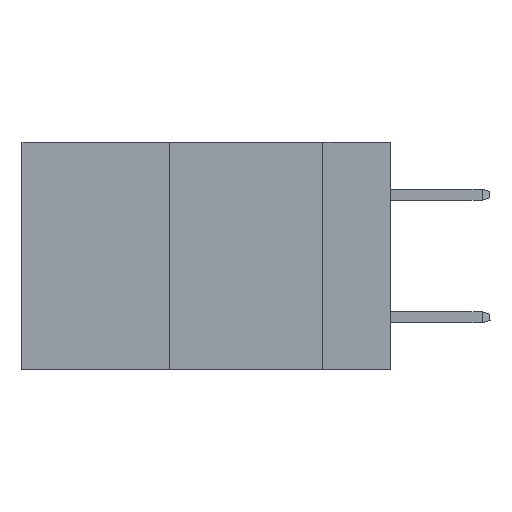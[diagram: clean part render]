
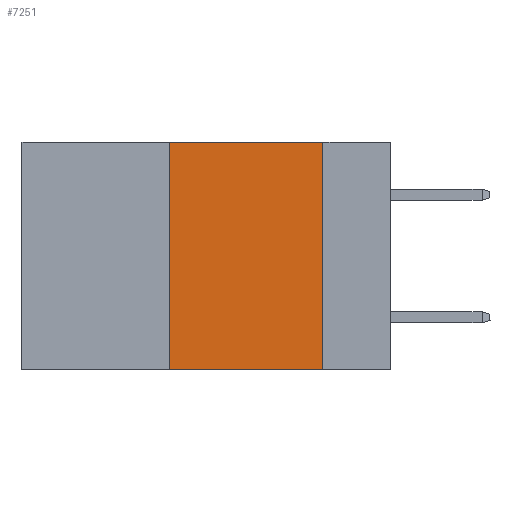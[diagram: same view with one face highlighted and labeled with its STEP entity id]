
A CAD part, left-side view. The second image highlights one B-rep face of the part: STEP entity #7251.
In plain terms, the highlighted planar face has unit normal (-1, 0, 0).
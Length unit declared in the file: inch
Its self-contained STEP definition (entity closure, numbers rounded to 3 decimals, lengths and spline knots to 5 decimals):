
#447 = EDGE_CURVE ( 'NONE', #14915, #10181, #13544, .T. ) ;
#807 = CARTESIAN_POINT ( 'NONE',  ( 0., 0.6, 0. ) ) ;
#812 = DIRECTION ( 'NONE',  ( 0., -1., 0. ) ) ;
#2126 = EDGE_LOOP ( 'NONE', ( #3064, #16125, #18472, #8523 ) ) ;
#2224 = DIRECTION ( 'NONE',  ( 1., 0., 0. ) ) ;
#2589 = DIRECTION ( 'NONE',  ( 0., -1., 0. ) ) ;
#3034 = DIRECTION ( 'NONE',  ( 0., 0., -1. ) ) ;
#3064 = ORIENTED_EDGE ( 'NONE', *, *, #12816, .F. ) ;
#3486 = CARTESIAN_POINT ( 'NONE',  ( 0., 0.6, -0.37 ) ) ;
#3496 = VECTOR ( 'NONE', #16801, 39.37008 ) ;
#3546 = EDGE_CURVE ( 'NONE', #14915, #8277, #7589, .T. ) ;
#4422 = VECTOR ( 'NONE', #812, 39.37008 ) ;
#6439 = LINE ( 'NONE', #11709, #15015 ) ;
#6639 = CARTESIAN_POINT ( 'NONE',  ( 0., 0.36, 0. ) ) ;
#7251 = ADVANCED_FACE ( 'NONE', ( #9905 ), #12539, .F. ) ;
#7589 = LINE ( 'NONE', #13075, #3496 ) ;
#8277 = VERTEX_POINT ( 'NONE', #6639 ) ;
#8523 = ORIENTED_EDGE ( 'NONE', *, *, #447, .T. ) ;
#8949 = CARTESIAN_POINT ( 'NONE',  ( 0., 0.36, -0.37 ) ) ;
#9905 = FACE_OUTER_BOUND ( 'NONE', #2126, .T. ) ;
#10031 = VERTEX_POINT ( 'NONE', #13288 ) ;
#10181 = VERTEX_POINT ( 'NONE', #11339 ) ;
#10905 = CARTESIAN_POINT ( 'NONE',  ( 0., 0.6, 0. ) ) ;
#11339 = CARTESIAN_POINT ( 'NONE',  ( 0., 0.11, -0.37 ) ) ;
#11709 = CARTESIAN_POINT ( 'NONE',  ( 0., 0.11, 0. ) ) ;
#12322 = AXIS2_PLACEMENT_3D ( 'NONE', #10905, #2224, #14265 ) ;
#12539 = PLANE ( 'NONE',  #12322 ) ;
#12816 = EDGE_CURVE ( 'NONE', #10031, #10181, #6439, .T. ) ;
#13075 = CARTESIAN_POINT ( 'NONE',  ( 0., 0.36, 0. ) ) ;
#13288 = CARTESIAN_POINT ( 'NONE',  ( 0., 0.11, 0. ) ) ;
#13544 = LINE ( 'NONE', #3486, #4422 ) ;
#14265 = DIRECTION ( 'NONE',  ( 0., 0., -1. ) ) ;
#14915 = VERTEX_POINT ( 'NONE', #8949 ) ;
#15015 = VECTOR ( 'NONE', #3034, 39.37008 ) ;
#16125 = ORIENTED_EDGE ( 'NONE', *, *, #21322, .F. ) ;
#16801 = DIRECTION ( 'NONE',  ( 0., 0., 1. ) ) ;
#17476 = VECTOR ( 'NONE', #2589, 39.37008 ) ;
#17994 = LINE ( 'NONE', #807, #17476 ) ;
#18472 = ORIENTED_EDGE ( 'NONE', *, *, #3546, .F. ) ;
#21322 = EDGE_CURVE ( 'NONE', #8277, #10031, #17994, .T. ) ;
